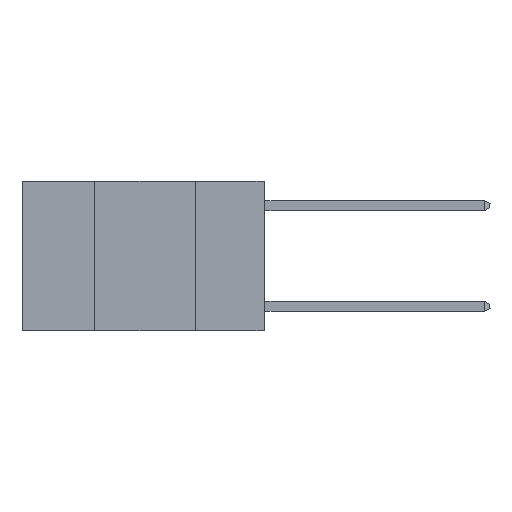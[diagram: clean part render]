
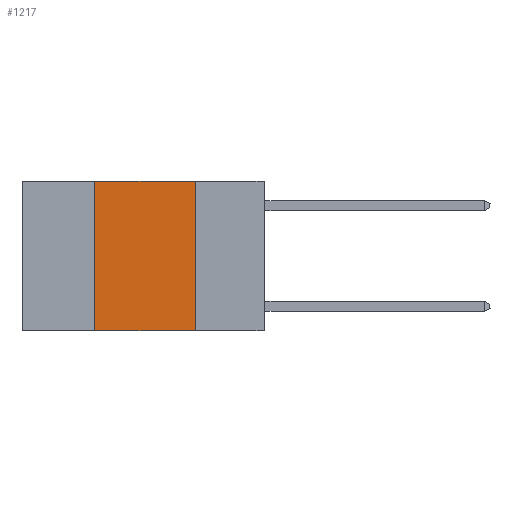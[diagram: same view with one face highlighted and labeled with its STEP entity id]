
A CAD part, left-side view. The second image highlights one B-rep face of the part: STEP entity #1217.
In plain terms, the highlighted planar face has unit normal (-1, 0, 0).
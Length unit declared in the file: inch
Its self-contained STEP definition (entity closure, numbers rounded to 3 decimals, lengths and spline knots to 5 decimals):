
#276 = LINE ( 'NONE', #3880, #5188 ) ;
#898 = EDGE_CURVE ( 'NONE', #11124, #7241, #8286, .T. ) ;
#1196 = AXIS2_PLACEMENT_3D ( 'NONE', #7543, #5505, #10297 ) ;
#1217 = ADVANCED_FACE ( 'NONE', ( #9062 ), #8148, .F. ) ;
#1763 = CARTESIAN_POINT ( 'NONE',  ( 0., 0.42, 0. ) ) ;
#1894 = EDGE_CURVE ( 'NONE', #4011, #7772, #276, .T. ) ;
#2026 = DIRECTION ( 'NONE',  ( 0., 0., -1. ) ) ;
#2366 = VECTOR ( 'NONE', #11181, 39.37008 ) ;
#3070 = CARTESIAN_POINT ( 'NONE',  ( 0., 0.42, -0.37 ) ) ;
#3104 = EDGE_CURVE ( 'NONE', #11124, #7772, #9535, .T. ) ;
#3880 = CARTESIAN_POINT ( 'NONE',  ( 0., 0.17, 0. ) ) ;
#4011 = VERTEX_POINT ( 'NONE', #8171 ) ;
#4218 = ORIENTED_EDGE ( 'NONE', *, *, #3104, .T. ) ;
#5188 = VECTOR ( 'NONE', #2026, 39.37008 ) ;
#5505 = DIRECTION ( 'NONE',  ( 1., 0., 0. ) ) ;
#5690 = ORIENTED_EDGE ( 'NONE', *, *, #10919, .F. ) ;
#5835 = CARTESIAN_POINT ( 'NONE',  ( 0., 0.6, -0.37 ) ) ;
#6703 = DIRECTION ( 'NONE',  ( 0., -1., 0. ) ) ;
#7241 = VERTEX_POINT ( 'NONE', #9776 ) ;
#7543 = CARTESIAN_POINT ( 'NONE',  ( 0., 0.6, 0. ) ) ;
#7772 = VERTEX_POINT ( 'NONE', #8006 ) ;
#7916 = VECTOR ( 'NONE', #6703, 39.37008 ) ;
#7950 = VECTOR ( 'NONE', #11874, 39.37008 ) ;
#7977 = EDGE_LOOP ( 'NONE', ( #11164, #5690, #11932, #4218 ) ) ;
#8006 = CARTESIAN_POINT ( 'NONE',  ( 0., 0.17, -0.37 ) ) ;
#8148 = PLANE ( 'NONE',  #1196 ) ;
#8171 = CARTESIAN_POINT ( 'NONE',  ( 0., 0.17, 0. ) ) ;
#8286 = LINE ( 'NONE', #1763, #2366 ) ;
#9062 = FACE_OUTER_BOUND ( 'NONE', #7977, .T. ) ;
#9535 = LINE ( 'NONE', #5835, #7916 ) ;
#9776 = CARTESIAN_POINT ( 'NONE',  ( 0., 0.42, 0. ) ) ;
#9972 = LINE ( 'NONE', #10830, #7950 ) ;
#10297 = DIRECTION ( 'NONE',  ( 0., 0., -1. ) ) ;
#10830 = CARTESIAN_POINT ( 'NONE',  ( 0., 0.6, 0. ) ) ;
#10919 = EDGE_CURVE ( 'NONE', #7241, #4011, #9972, .T. ) ;
#11124 = VERTEX_POINT ( 'NONE', #3070 ) ;
#11164 = ORIENTED_EDGE ( 'NONE', *, *, #1894, .F. ) ;
#11181 = DIRECTION ( 'NONE',  ( 0., 0., 1. ) ) ;
#11874 = DIRECTION ( 'NONE',  ( 0., -1., 0. ) ) ;
#11932 = ORIENTED_EDGE ( 'NONE', *, *, #898, .F. ) ;
